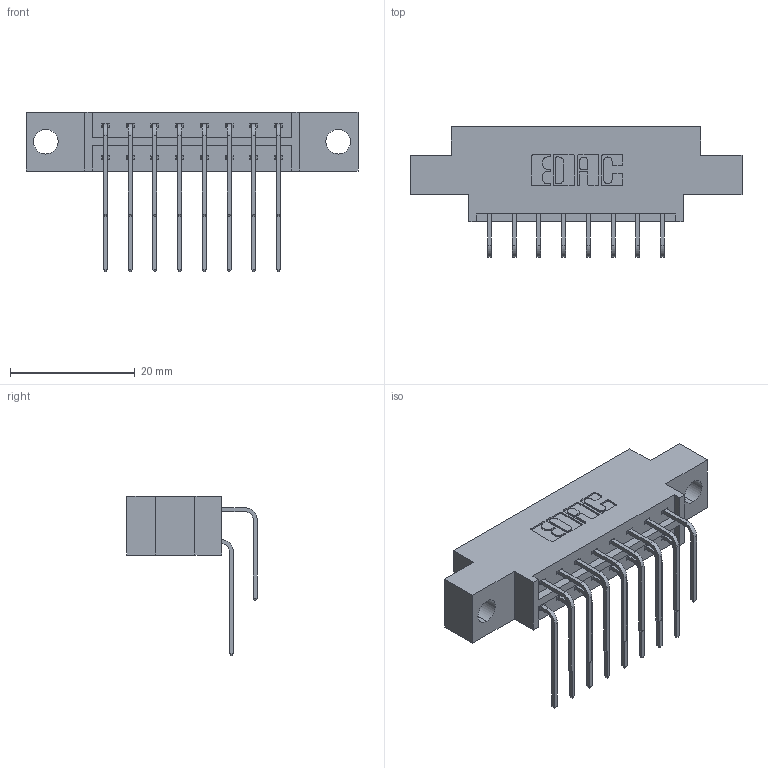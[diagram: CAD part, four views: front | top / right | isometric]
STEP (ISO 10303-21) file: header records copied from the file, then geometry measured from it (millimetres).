
FILE_DESCRIPTION (( 'STEP AP203' ), '1' );
FILE_NAME ('833-016-559-804.STEP', '2020-05-31T19:15:50', ( '' ), ( '' ), 'SwSTEP 2.0', 'SolidWorks 2020', '' );
FILE_SCHEMA (( 'CONFIG_CONTROL_DESIGN' ));
Length unit declared in the file: inch
Products named in the file (4): 833-016-559-804; 833 Part_Offset - .156 Dia - TH; 345-292-001_559 Tail - 2; 345-292-001_558 559 Tail - 1
Assembly tree (17 placements, depth 2):
  833-016-559-804
    833 Part_Offset - .156 Dia - TH
    345-292-001_558 559 Tail - 1  x8
    345-292-001_559 Tail - 2  x8
Bounding box: 53.24 x 20.9 x 25.53 mm (x, y, z)
Volume: 4894 mm3; surface area: 5900.6 mm2
Topology: 17 solids, 17 shells, 982 faces, 2899 edges, 1910 vertices
Faces by surface type: plane 682, cylinder 300
Entity records: 11463 total; most frequent: CARTESIAN_POINT 1993, ORIENTED_EDGE 1878, DIRECTION 1743, EDGE_CURVE 939, LINE 771, VECTOR 771, VERTEX_POINT 622, AXIS2_PLACEMENT_3D 486
